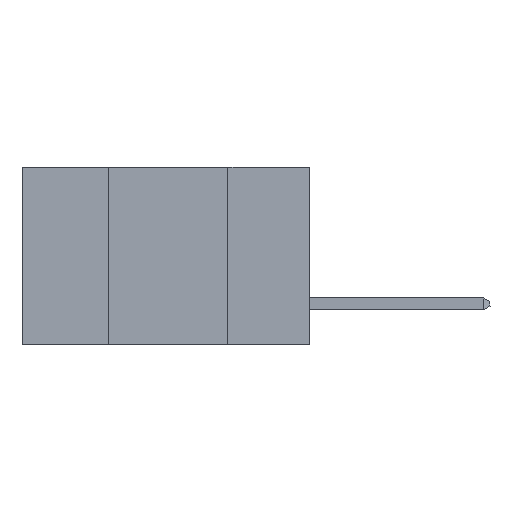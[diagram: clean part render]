
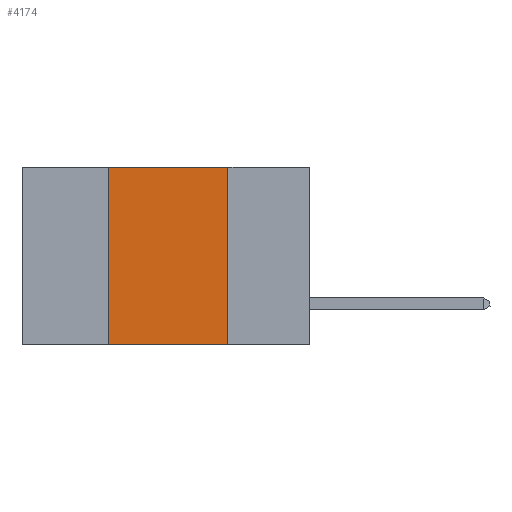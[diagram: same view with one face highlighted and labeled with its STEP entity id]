
A CAD part, left-side view. The second image highlights one B-rep face of the part: STEP entity #4174.
In plain terms, the highlighted planar face has unit normal (-1, 0, 0).
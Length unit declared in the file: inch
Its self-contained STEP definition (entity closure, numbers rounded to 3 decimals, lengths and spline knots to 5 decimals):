
#286 = AXIS2_PLACEMENT_3D ( 'NONE', #533, #2960, #2992 ) ;
#533 = CARTESIAN_POINT ( 'NONE',  ( 0., 0.6, 0. ) ) ;
#736 = PLANE ( 'NONE',  #286 ) ;
#1421 = EDGE_CURVE ( 'NONE', #11027, #3430, #5580, .T. ) ;
#1908 = DIRECTION ( 'NONE',  ( 0., 0., -1. ) ) ;
#2368 = VERTEX_POINT ( 'NONE', #17005 ) ;
#2960 = DIRECTION ( 'NONE',  ( 1., 0., 0. ) ) ;
#2992 = DIRECTION ( 'NONE',  ( 0., 0., -1. ) ) ;
#3430 = VERTEX_POINT ( 'NONE', #14398 ) ;
#4174 = ADVANCED_FACE ( 'NONE', ( #6630 ), #736, .F. ) ;
#5181 = VERTEX_POINT ( 'NONE', #7586 ) ;
#5580 = LINE ( 'NONE', #12869, #8791 ) ;
#5746 = EDGE_LOOP ( 'NONE', ( #16000, #12392, #12377, #11054 ) ) ;
#5988 = DIRECTION ( 'NONE',  ( 0., 0., 1. ) ) ;
#6337 = CARTESIAN_POINT ( 'NONE',  ( 0., 0.6, 0. ) ) ;
#6376 = VECTOR ( 'NONE', #16480, 39.37008 ) ;
#6552 = CARTESIAN_POINT ( 'NONE',  ( 0., 0.17, 0. ) ) ;
#6630 = FACE_OUTER_BOUND ( 'NONE', #5746, .T. ) ;
#6876 = LINE ( 'NONE', #6337, #13555 ) ;
#7586 = CARTESIAN_POINT ( 'NONE',  ( 0., 0.17, 0. ) ) ;
#7599 = EDGE_CURVE ( 'NONE', #5181, #2368, #11320, .T. ) ;
#7783 = VECTOR ( 'NONE', #1908, 39.37008 ) ;
#8791 = VECTOR ( 'NONE', #5988, 39.37008 ) ;
#9958 = CARTESIAN_POINT ( 'NONE',  ( 0., 0.6, -0.37 ) ) ;
#11027 = VERTEX_POINT ( 'NONE', #12424 ) ;
#11054 = ORIENTED_EDGE ( 'NONE', *, *, #14262, .T. ) ;
#11320 = LINE ( 'NONE', #6552, #7783 ) ;
#12377 = ORIENTED_EDGE ( 'NONE', *, *, #1421, .F. ) ;
#12392 = ORIENTED_EDGE ( 'NONE', *, *, #12584, .F. ) ;
#12424 = CARTESIAN_POINT ( 'NONE',  ( 0., 0.42, -0.37 ) ) ;
#12584 = EDGE_CURVE ( 'NONE', #3430, #5181, #6876, .T. ) ;
#12869 = CARTESIAN_POINT ( 'NONE',  ( 0., 0.42, 0. ) ) ;
#13555 = VECTOR ( 'NONE', #16898, 39.37008 ) ;
#14262 = EDGE_CURVE ( 'NONE', #11027, #2368, #17298, .T. ) ;
#14398 = CARTESIAN_POINT ( 'NONE',  ( 0., 0.42, 0. ) ) ;
#16000 = ORIENTED_EDGE ( 'NONE', *, *, #7599, .F. ) ;
#16480 = DIRECTION ( 'NONE',  ( 0., -1., 0. ) ) ;
#16898 = DIRECTION ( 'NONE',  ( 0., -1., 0. ) ) ;
#17005 = CARTESIAN_POINT ( 'NONE',  ( 0., 0.17, -0.37 ) ) ;
#17298 = LINE ( 'NONE', #9958, #6376 ) ;
